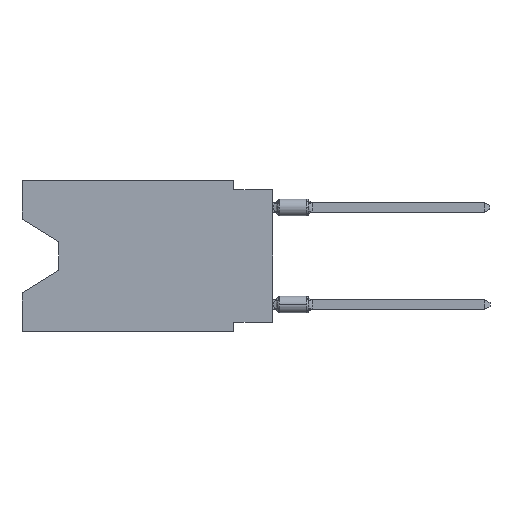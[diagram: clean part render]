
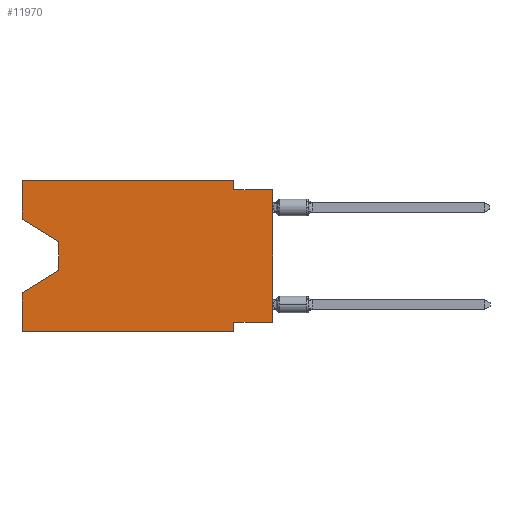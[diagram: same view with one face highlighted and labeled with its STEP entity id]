
A CAD part, left-side view. The second image highlights one B-rep face of the part: STEP entity #11970.
In plain terms, the highlighted planar face has unit normal (-1, 0, 0).
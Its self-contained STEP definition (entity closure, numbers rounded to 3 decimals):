
#126 = EDGE_CURVE ( 'NONE', #10238, #16141, #12757, .T. ) ;
#339 = CARTESIAN_POINT ( 'NONE',  ( 0., 13.97, -4.013 ) ) ;
#485 = ORIENTED_EDGE ( 'NONE', *, *, #8935, .T. ) ;
#514 = VECTOR ( 'NONE', #3277, 1000. ) ;
#611 = VECTOR ( 'NONE', #10551, 1000. ) ;
#819 = VECTOR ( 'NONE', #13959, 1000. ) ;
#1099 = VERTEX_POINT ( 'NONE', #2931 ) ;
#1121 = CARTESIAN_POINT ( 'NONE',  ( 0., 2.54, -0.635 ) ) ;
#1142 = CARTESIAN_POINT ( 'NONE',  ( 0., 0., -0.635 ) ) ;
#1297 = DIRECTION ( 'NONE',  ( 0., 0., -1. ) ) ;
#1375 = FACE_OUTER_BOUND ( 'NONE', #14823, .T. ) ;
#1808 = CARTESIAN_POINT ( 'NONE',  ( 0., 0., -0.635 ) ) ;
#2241 = CARTESIAN_POINT ( 'NONE',  ( 0., 13.97, -5.893 ) ) ;
#2298 = EDGE_CURVE ( 'NONE', #15585, #11580, #14782, .T. ) ;
#2363 = DIRECTION ( 'NONE',  ( 0., 0., 1. ) ) ;
#2412 = VECTOR ( 'NONE', #5026, 1000. ) ;
#2755 = CARTESIAN_POINT ( 'NONE',  ( 0., 16.383, 0. ) ) ;
#2882 = CARTESIAN_POINT ( 'NONE',  ( 0., 16.383, 0. ) ) ;
#2929 = DIRECTION ( 'NONE',  ( 1., 0., 0. ) ) ;
#2931 = CARTESIAN_POINT ( 'NONE',  ( 0., 16.383, -7.36 ) ) ;
#3138 = CARTESIAN_POINT ( 'NONE',  ( 0., 13.97, -4.013 ) ) ;
#3249 = VERTEX_POINT ( 'NONE', #8420 ) ;
#3277 = DIRECTION ( 'NONE',  ( 0., -1., 0. ) ) ;
#3386 = EDGE_CURVE ( 'NONE', #3249, #15585, #10006, .T. ) ;
#3390 = LINE ( 'NONE', #13687, #6423 ) ;
#3469 = DIRECTION ( 'NONE',  ( 0., 0., -1. ) ) ;
#3666 = CARTESIAN_POINT ( 'NONE',  ( 0., 16.383, 0. ) ) ;
#3846 = ORIENTED_EDGE ( 'NONE', *, *, #13245, .F. ) ;
#4210 = EDGE_CURVE ( 'NONE', #11151, #1099, #11737, .T. ) ;
#4339 = LINE ( 'NONE', #339, #15309 ) ;
#4384 = ORIENTED_EDGE ( 'NONE', *, *, #2298, .F. ) ;
#4475 = CARTESIAN_POINT ( 'NONE',  ( 0., 0., -9.271 ) ) ;
#4925 = EDGE_CURVE ( 'NONE', #13602, #14820, #15176, .T. ) ;
#4940 = ORIENTED_EDGE ( 'NONE', *, *, #10752, .T. ) ;
#4973 = CARTESIAN_POINT ( 'NONE',  ( 0., 16.383, -9.906 ) ) ;
#5026 = DIRECTION ( 'NONE',  ( 0., 0.855, -0.519 ) ) ;
#5624 = DIRECTION ( 'NONE',  ( 0., 0., -1. ) ) ;
#6081 = CARTESIAN_POINT ( 'NONE',  ( 0., 2.54, 0. ) ) ;
#6240 = VECTOR ( 'NONE', #13973, 1000. ) ;
#6311 = ORIENTED_EDGE ( 'NONE', *, *, #14077, .F. ) ;
#6400 = CARTESIAN_POINT ( 'NONE',  ( 0., 2.54, -9.906 ) ) ;
#6423 = VECTOR ( 'NONE', #8689, 1000. ) ;
#6583 = VERTEX_POINT ( 'NONE', #3138 ) ;
#7269 = LINE ( 'NONE', #11383, #514 ) ;
#7351 = ORIENTED_EDGE ( 'NONE', *, *, #15278, .F. ) ;
#7364 = CARTESIAN_POINT ( 'NONE',  ( 0., 16.383, -9.906 ) ) ;
#7473 = ORIENTED_EDGE ( 'NONE', *, *, #10631, .T. ) ;
#8017 = VERTEX_POINT ( 'NONE', #6400 ) ;
#8029 = ORIENTED_EDGE ( 'NONE', *, *, #4210, .T. ) ;
#8420 = CARTESIAN_POINT ( 'NONE',  ( 0., 2.54, 0. ) ) ;
#8663 = DIRECTION ( 'NONE',  ( 0., -1., 0. ) ) ;
#8689 = DIRECTION ( 'NONE',  ( 0., 0., 1. ) ) ;
#8702 = LINE ( 'NONE', #9196, #819 ) ;
#8731 = CARTESIAN_POINT ( 'NONE',  ( 0., 13.97, -5.893 ) ) ;
#8935 = EDGE_CURVE ( 'NONE', #10238, #6583, #11943, .T. ) ;
#8970 = CARTESIAN_POINT ( 'NONE',  ( 0., 16.383, 0. ) ) ;
#9196 = CARTESIAN_POINT ( 'NONE',  ( 0., 2.54, -9.906 ) ) ;
#9820 = VECTOR ( 'NONE', #2363, 1000. ) ;
#10006 = LINE ( 'NONE', #6081, #12127 ) ;
#10238 = VERTEX_POINT ( 'NONE', #11234 ) ;
#10291 = LINE ( 'NONE', #3666, #17148 ) ;
#10464 = ORIENTED_EDGE ( 'NONE', *, *, #3386, .F. ) ;
#10551 = DIRECTION ( 'NONE',  ( 0., -0.855, -0.519 ) ) ;
#10631 = EDGE_CURVE ( 'NONE', #6583, #11151, #4339, .T. ) ;
#10722 = VECTOR ( 'NONE', #10864, 1000. ) ;
#10752 = EDGE_CURVE ( 'NONE', #12654, #8017, #15383, .T. ) ;
#10864 = DIRECTION ( 'NONE',  ( 0., -1., 0. ) ) ;
#10888 = CARTESIAN_POINT ( 'NONE',  ( 0., 16.383, -2.546 ) ) ;
#11151 = VERTEX_POINT ( 'NONE', #8731 ) ;
#11234 = CARTESIAN_POINT ( 'NONE',  ( 0., 16.383, -2.546 ) ) ;
#11383 = CARTESIAN_POINT ( 'NONE',  ( 0., 16.383, 0. ) ) ;
#11412 = EDGE_CURVE ( 'NONE', #13602, #11580, #3390, .T. ) ;
#11446 = AXIS2_PLACEMENT_3D ( 'NONE', #2755, #2929, #1297 ) ;
#11515 = DIRECTION ( 'NONE',  ( 0., 0., 1. ) ) ;
#11580 = VERTEX_POINT ( 'NONE', #1142 ) ;
#11737 = LINE ( 'NONE', #2241, #2412 ) ;
#11800 = ORIENTED_EDGE ( 'NONE', *, *, #126, .F. ) ;
#11943 = LINE ( 'NONE', #10888, #611 ) ;
#11970 = ADVANCED_FACE ( 'NONE', ( #1375 ), #12084, .F. ) ;
#12084 = PLANE ( 'NONE',  #11446 ) ;
#12127 = VECTOR ( 'NONE', #3469, 1000. ) ;
#12654 = VERTEX_POINT ( 'NONE', #4973 ) ;
#12757 = LINE ( 'NONE', #8970, #9820 ) ;
#13097 = ORIENTED_EDGE ( 'NONE', *, *, #11412, .T. ) ;
#13245 = EDGE_CURVE ( 'NONE', #16141, #3249, #7269, .T. ) ;
#13602 = VERTEX_POINT ( 'NONE', #4475 ) ;
#13687 = CARTESIAN_POINT ( 'NONE',  ( 0., 0., 0. ) ) ;
#13892 = CARTESIAN_POINT ( 'NONE',  ( 0., 0., -9.271 ) ) ;
#13959 = DIRECTION ( 'NONE',  ( 0., 0., -1. ) ) ;
#13973 = DIRECTION ( 'NONE',  ( 0., 1., 0. ) ) ;
#14077 = EDGE_CURVE ( 'NONE', #14820, #8017, #8702, .T. ) ;
#14782 = LINE ( 'NONE', #1808, #10722 ) ;
#14820 = VERTEX_POINT ( 'NONE', #16400 ) ;
#14823 = EDGE_LOOP ( 'NONE', ( #485, #7473, #8029, #7351, #4940, #6311, #16553, #13097, #4384, #10464, #3846, #11800 ) ) ;
#15176 = LINE ( 'NONE', #13892, #6240 ) ;
#15278 = EDGE_CURVE ( 'NONE', #12654, #1099, #10291, .T. ) ;
#15309 = VECTOR ( 'NONE', #5624, 1000. ) ;
#15383 = LINE ( 'NONE', #7364, #16138 ) ;
#15585 = VERTEX_POINT ( 'NONE', #1121 ) ;
#16138 = VECTOR ( 'NONE', #8663, 1000. ) ;
#16141 = VERTEX_POINT ( 'NONE', #2882 ) ;
#16400 = CARTESIAN_POINT ( 'NONE',  ( 0., 2.54, -9.271 ) ) ;
#16553 = ORIENTED_EDGE ( 'NONE', *, *, #4925, .F. ) ;
#17148 = VECTOR ( 'NONE', #11515, 1000. ) ;
